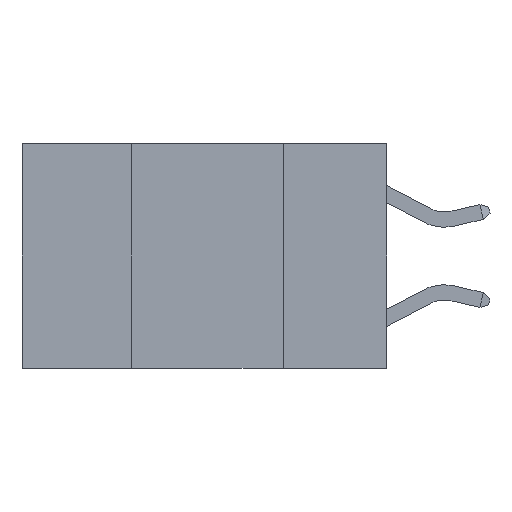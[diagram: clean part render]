
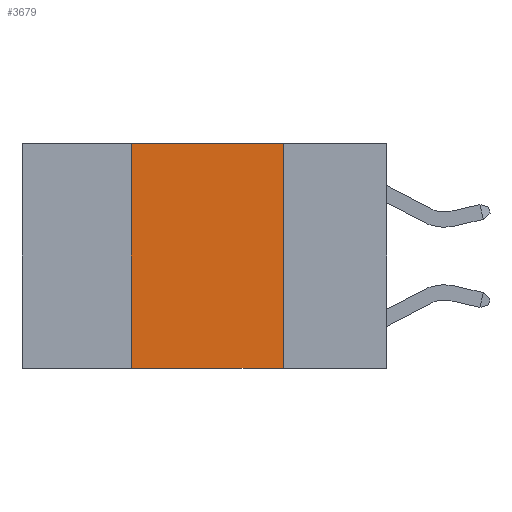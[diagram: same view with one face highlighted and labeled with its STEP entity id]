
A CAD part, left-side view. The second image highlights one B-rep face of the part: STEP entity #3679.
In plain terms, the highlighted planar face has unit normal (-1, 0, 0).
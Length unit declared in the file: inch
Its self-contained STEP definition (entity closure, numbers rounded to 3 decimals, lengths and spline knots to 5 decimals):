
#24 = ORIENTED_EDGE ( 'NONE', *, *, #11152, .T. ) ;
#874 = CARTESIAN_POINT ( 'NONE',  ( 0., 0.6, 0. ) ) ;
#1506 = DIRECTION ( 'NONE',  ( 1., 0., 0. ) ) ;
#1757 = CARTESIAN_POINT ( 'NONE',  ( 0., 0.6, -0.37 ) ) ;
#1771 = EDGE_CURVE ( 'NONE', #5746, #10144, #5020, .T. ) ;
#2245 = DIRECTION ( 'NONE',  ( 0., 0., 1. ) ) ;
#2288 = CARTESIAN_POINT ( 'NONE',  ( 0., 0.42, 0. ) ) ;
#2648 = CARTESIAN_POINT ( 'NONE',  ( 0., 0.17, 0. ) ) ;
#2695 = DIRECTION ( 'NONE',  ( 0., -1., 0. ) ) ;
#2721 = FACE_OUTER_BOUND ( 'NONE', #4710, .T. ) ;
#2733 = EDGE_CURVE ( 'NONE', #10144, #5768, #5592, .T. ) ;
#2768 = VECTOR ( 'NONE', #2245, 39.37008 ) ;
#3172 = CARTESIAN_POINT ( 'NONE',  ( 0., 0.42, 0. ) ) ;
#3187 = AXIS2_PLACEMENT_3D ( 'NONE', #3393, #1506, #8184 ) ;
#3393 = CARTESIAN_POINT ( 'NONE',  ( 0., 0.6, 0. ) ) ;
#3679 = ADVANCED_FACE ( 'NONE', ( #2721 ), #7246, .F. ) ;
#4075 = ORIENTED_EDGE ( 'NONE', *, *, #1771, .F. ) ;
#4710 = EDGE_LOOP ( 'NONE', ( #6441, #12296, #4075, #24 ) ) ;
#4818 = CARTESIAN_POINT ( 'NONE',  ( 0., 0.17, -0.37 ) ) ;
#5020 = LINE ( 'NONE', #2288, #2768 ) ;
#5297 = VECTOR ( 'NONE', #5667, 39.37008 ) ;
#5592 = LINE ( 'NONE', #874, #5297 ) ;
#5667 = DIRECTION ( 'NONE',  ( 0., -1., 0. ) ) ;
#5746 = VERTEX_POINT ( 'NONE', #12199 ) ;
#5768 = VERTEX_POINT ( 'NONE', #2648 ) ;
#6441 = ORIENTED_EDGE ( 'NONE', *, *, #12271, .F. ) ;
#7246 = PLANE ( 'NONE',  #3187 ) ;
#8184 = DIRECTION ( 'NONE',  ( 0., 0., -1. ) ) ;
#8692 = VECTOR ( 'NONE', #2695, 39.37008 ) ;
#9004 = LINE ( 'NONE', #1757, #8692 ) ;
#9225 = CARTESIAN_POINT ( 'NONE',  ( 0., 0.17, 0. ) ) ;
#9411 = LINE ( 'NONE', #9225, #11626 ) ;
#9925 = VERTEX_POINT ( 'NONE', #4818 ) ;
#10144 = VERTEX_POINT ( 'NONE', #3172 ) ;
#10171 = DIRECTION ( 'NONE',  ( 0., 0., -1. ) ) ;
#11152 = EDGE_CURVE ( 'NONE', #5746, #9925, #9004, .T. ) ;
#11626 = VECTOR ( 'NONE', #10171, 39.37008 ) ;
#12199 = CARTESIAN_POINT ( 'NONE',  ( 0., 0.42, -0.37 ) ) ;
#12271 = EDGE_CURVE ( 'NONE', #5768, #9925, #9411, .T. ) ;
#12296 = ORIENTED_EDGE ( 'NONE', *, *, #2733, .F. ) ;
